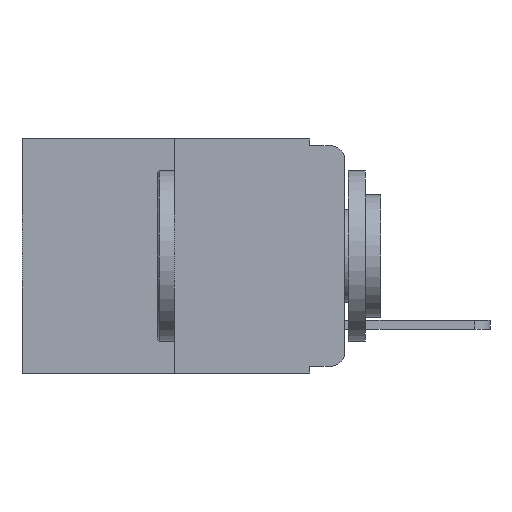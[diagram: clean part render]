
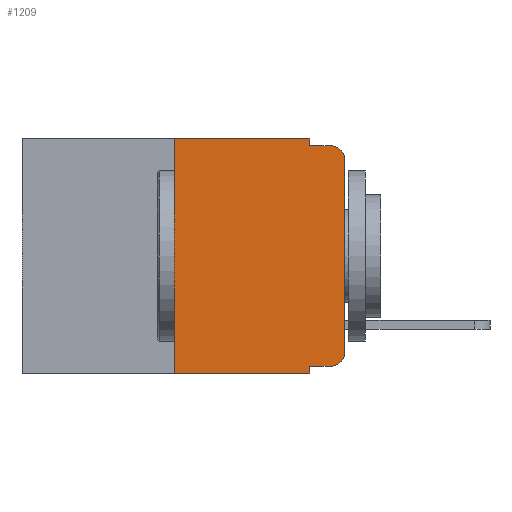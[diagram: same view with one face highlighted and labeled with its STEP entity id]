
A CAD part, left-side view. The second image highlights one B-rep face of the part: STEP entity #1209.
In plain terms, the highlighted planar face has unit normal (-1, 0, 0).
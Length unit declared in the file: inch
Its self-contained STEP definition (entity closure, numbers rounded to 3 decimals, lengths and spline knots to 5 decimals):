
#79 = EDGE_LOOP ( 'NONE', ( #7748, #7271, #6753, #6627, #5991, #5522, #4659, #3325, #5261, #4197 ) ) ;
#86 = EDGE_CURVE ( 'NONE', #10736, #4881, #2221, .T. ) ;
#102 = CIRCLE ( 'NONE', #3823, 0.02 ) ;
#138 = DIRECTION ( 'NONE',  ( 0., 0., 1. ) ) ;
#195 = EDGE_CURVE ( 'NONE', #4881, #3002, #8755, .T. ) ;
#253 = EDGE_CURVE ( 'NONE', #9055, #5234, #5122, .T. ) ;
#306 = DIRECTION ( 'NONE',  ( 1., 0., 0. ) ) ;
#336 = LINE ( 'NONE', #4215, #3588 ) ;
#452 = VERTEX_POINT ( 'NONE', #6401 ) ;
#490 = CARTESIAN_POINT ( 'NONE',  ( 0., 0.051, -0.01 ) ) ;
#842 = VECTOR ( 'NONE', #5188, 39.37008 ) ;
#937 = EDGE_CURVE ( 'NONE', #9658, #3002, #11640, .T. ) ;
#1010 = CARTESIAN_POINT ( 'NONE',  ( 0., 0.02, -0.03 ) ) ;
#1159 = EDGE_CURVE ( 'NONE', #5234, #452, #102, .T. ) ;
#1209 = ADVANCED_FACE ( 'NONE', ( #5434 ), #3694, .F. ) ;
#1224 = EDGE_CURVE ( 'NONE', #452, #9658, #10537, .T. ) ;
#1897 = VERTEX_POINT ( 'NONE', #7955 ) ;
#1973 = DIRECTION ( 'NONE',  ( 0., 0., -1. ) ) ;
#1988 = DIRECTION ( 'NONE',  ( -1., 0., 0. ) ) ;
#2221 = LINE ( 'NONE', #8881, #12689 ) ;
#2299 = VERTEX_POINT ( 'NONE', #11480 ) ;
#3002 = VERTEX_POINT ( 'NONE', #12423 ) ;
#3200 = CARTESIAN_POINT ( 'NONE',  ( 0., 0.25, 0. ) ) ;
#3325 = ORIENTED_EDGE ( 'NONE', *, *, #6680, .F. ) ;
#3588 = VECTOR ( 'NONE', #4154, 39.37008 ) ;
#3694 = PLANE ( 'NONE',  #7154 ) ;
#3701 = DIRECTION ( 'NONE',  ( 0., -1., 0. ) ) ;
#3717 = VECTOR ( 'NONE', #10117, 39.37008 ) ;
#3756 = LINE ( 'NONE', #11366, #842 ) ;
#3823 = AXIS2_PLACEMENT_3D ( 'NONE', #11383, #6288, #7673 ) ;
#4058 = CARTESIAN_POINT ( 'NONE',  ( 0., 0.473, 0. ) ) ;
#4119 = CARTESIAN_POINT ( 'NONE',  ( 0., 0., -0.03 ) ) ;
#4154 = DIRECTION ( 'NONE',  ( 0., 0., -1. ) ) ;
#4197 = ORIENTED_EDGE ( 'NONE', *, *, #1159, .T. ) ;
#4215 = CARTESIAN_POINT ( 'NONE',  ( 0., 0.051, 0. ) ) ;
#4659 = ORIENTED_EDGE ( 'NONE', *, *, #6317, .T. ) ;
#4881 = VERTEX_POINT ( 'NONE', #490 ) ;
#5025 = DIRECTION ( 'NONE',  ( 0., 0., -1. ) ) ;
#5122 = LINE ( 'NONE', #10836, #7794 ) ;
#5146 = VERTEX_POINT ( 'NONE', #10294 ) ;
#5188 = DIRECTION ( 'NONE',  ( 0., -1., 0. ) ) ;
#5234 = VERTEX_POINT ( 'NONE', #9938 ) ;
#5261 = ORIENTED_EDGE ( 'NONE', *, *, #253, .T. ) ;
#5434 = FACE_OUTER_BOUND ( 'NONE', #79, .T. ) ;
#5522 = ORIENTED_EDGE ( 'NONE', *, *, #6433, .F. ) ;
#5784 = VECTOR ( 'NONE', #138, 39.37008 ) ;
#5791 = CARTESIAN_POINT ( 'NONE',  ( 0., 0.473, 0. ) ) ;
#5991 = ORIENTED_EDGE ( 'NONE', *, *, #8092, .F. ) ;
#6110 = CARTESIAN_POINT ( 'NONE',  ( 0., 0., 0. ) ) ;
#6127 = DIRECTION ( 'NONE',  ( 0., 0., 1. ) ) ;
#6288 = DIRECTION ( 'NONE',  ( -1., 0., 0. ) ) ;
#6317 = EDGE_CURVE ( 'NONE', #1897, #2299, #3756, .T. ) ;
#6401 = CARTESIAN_POINT ( 'NONE',  ( 0., 0., -0.313 ) ) ;
#6433 = EDGE_CURVE ( 'NONE', #1897, #5146, #11208, .T. ) ;
#6627 = ORIENTED_EDGE ( 'NONE', *, *, #86, .F. ) ;
#6680 = EDGE_CURVE ( 'NONE', #9055, #2299, #336, .T. ) ;
#6753 = ORIENTED_EDGE ( 'NONE', *, *, #195, .F. ) ;
#7154 = AXIS2_PLACEMENT_3D ( 'NONE', #5791, #306, #5025 ) ;
#7271 = ORIENTED_EDGE ( 'NONE', *, *, #937, .T. ) ;
#7673 = DIRECTION ( 'NONE',  ( 0., 0., -1. ) ) ;
#7748 = ORIENTED_EDGE ( 'NONE', *, *, #1224, .T. ) ;
#7784 = VECTOR ( 'NONE', #6127, 39.37008 ) ;
#7794 = VECTOR ( 'NONE', #10822, 39.37008 ) ;
#7841 = DIRECTION ( 'NONE',  ( 0., 0., -1. ) ) ;
#7955 = CARTESIAN_POINT ( 'NONE',  ( 0., 0.25, -0.343 ) ) ;
#8092 = EDGE_CURVE ( 'NONE', #5146, #10736, #11934, .T. ) ;
#8755 = LINE ( 'NONE', #10076, #3717 ) ;
#8881 = CARTESIAN_POINT ( 'NONE',  ( 0., 0.051, 0. ) ) ;
#9043 = AXIS2_PLACEMENT_3D ( 'NONE', #1010, #1988, #1973 ) ;
#9055 = VERTEX_POINT ( 'NONE', #11335 ) ;
#9078 = CARTESIAN_POINT ( 'NONE',  ( 0., 0.051, 0. ) ) ;
#9226 = VECTOR ( 'NONE', #3701, 39.37008 ) ;
#9658 = VERTEX_POINT ( 'NONE', #4119 ) ;
#9938 = CARTESIAN_POINT ( 'NONE',  ( 0., 0.02, -0.333 ) ) ;
#10076 = CARTESIAN_POINT ( 'NONE',  ( 0., 0.051, -0.01 ) ) ;
#10117 = DIRECTION ( 'NONE',  ( 0., -1., 0. ) ) ;
#10294 = CARTESIAN_POINT ( 'NONE',  ( 0., 0.25, 0. ) ) ;
#10537 = LINE ( 'NONE', #6110, #7784 ) ;
#10736 = VERTEX_POINT ( 'NONE', #9078 ) ;
#10822 = DIRECTION ( 'NONE',  ( 0., -1., 0. ) ) ;
#10836 = CARTESIAN_POINT ( 'NONE',  ( 0., 0.051, -0.333 ) ) ;
#11208 = LINE ( 'NONE', #3200, #5784 ) ;
#11335 = CARTESIAN_POINT ( 'NONE',  ( 0., 0.051, -0.333 ) ) ;
#11366 = CARTESIAN_POINT ( 'NONE',  ( 0., 0.473, -0.343 ) ) ;
#11383 = CARTESIAN_POINT ( 'NONE',  ( 0., 0.02, -0.313 ) ) ;
#11480 = CARTESIAN_POINT ( 'NONE',  ( 0., 0.051, -0.343 ) ) ;
#11640 = CIRCLE ( 'NONE', #9043, 0.02 ) ;
#11934 = LINE ( 'NONE', #4058, #9226 ) ;
#12423 = CARTESIAN_POINT ( 'NONE',  ( 0., 0.02, -0.01 ) ) ;
#12689 = VECTOR ( 'NONE', #7841, 39.37008 ) ;
